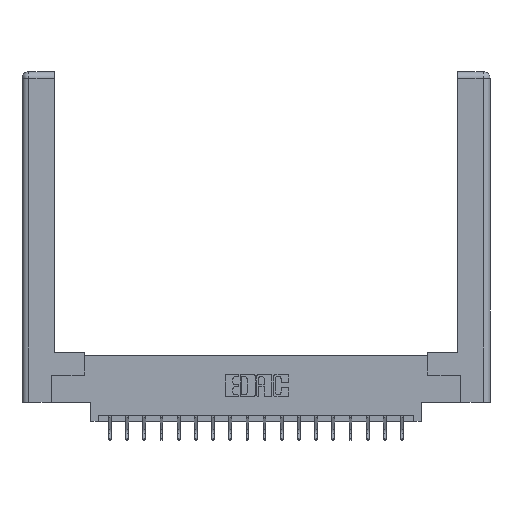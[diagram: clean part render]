
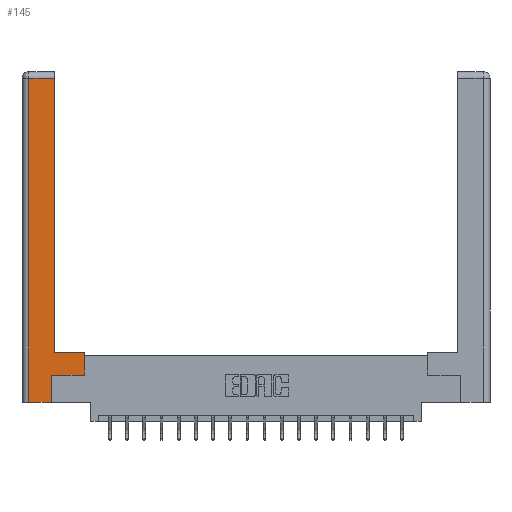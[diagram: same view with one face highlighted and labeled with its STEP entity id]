
A CAD part, top view. The second image highlights one B-rep face of the part: STEP entity #145.
In plain terms, the highlighted planar face has unit normal (0, 0, 1).
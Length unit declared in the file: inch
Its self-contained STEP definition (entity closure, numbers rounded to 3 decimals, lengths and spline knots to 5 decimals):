
#145 = ADVANCED_FACE ( 'NONE', ( #19700 ), #7569, .F. ) ;
#314 = CARTESIAN_POINT ( 'NONE',  ( 0.565, 0.245, 0. ) ) ;
#744 = VECTOR ( 'NONE', #5296, 39.37008 ) ;
#843 = CARTESIAN_POINT ( 'NONE',  ( 0.265, 0., 0. ) ) ;
#1026 = VERTEX_POINT ( 'NONE', #8673 ) ;
#1340 = LINE ( 'NONE', #14225, #16392 ) ;
#1631 = CARTESIAN_POINT ( 'NONE',  ( 0.0615, 2.94, 0. ) ) ;
#2412 = EDGE_CURVE ( 'NONE', #9835, #17495, #4857, .T. ) ;
#2894 = EDGE_CURVE ( 'NONE', #1026, #15038, #7751, .T. ) ;
#3127 = DIRECTION ( 'NONE',  ( -1., 0., 0. ) ) ;
#3463 = CARTESIAN_POINT ( 'NONE',  ( 0.295, 3., 0. ) ) ;
#3524 = DIRECTION ( 'NONE',  ( -1., 0., 0. ) ) ;
#3970 = ORIENTED_EDGE ( 'NONE', *, *, #2412, .T. ) ;
#4178 = ORIENTED_EDGE ( 'NONE', *, *, #19237, .T. ) ;
#4364 = ORIENTED_EDGE ( 'NONE', *, *, #2894, .T. ) ;
#4411 = DIRECTION ( 'NONE',  ( -1., 0., 0. ) ) ;
#4857 = LINE ( 'NONE', #3463, #7535 ) ;
#5009 = ORIENTED_EDGE ( 'NONE', *, *, #16505, .T. ) ;
#5290 = VERTEX_POINT ( 'NONE', #843 ) ;
#5296 = DIRECTION ( 'NONE',  ( 0., -1., 0. ) ) ;
#6194 = ORIENTED_EDGE ( 'NONE', *, *, #15344, .T. ) ;
#6215 = VECTOR ( 'NONE', #14056, 39.37008 ) ;
#6454 = CARTESIAN_POINT ( 'NONE',  ( 0.295, 0.45, 0. ) ) ;
#7167 = ORIENTED_EDGE ( 'NONE', *, *, #18820, .T. ) ;
#7535 = VECTOR ( 'NONE', #15695, 39.37008 ) ;
#7569 = PLANE ( 'NONE',  #8427 ) ;
#7751 = LINE ( 'NONE', #314, #10920 ) ;
#7801 = CARTESIAN_POINT ( 'NONE',  ( 0.265, 0., 0. ) ) ;
#7970 = CARTESIAN_POINT ( 'NONE',  ( 0.565, 0.245, 0. ) ) ;
#8125 = CARTESIAN_POINT ( 'NONE',  ( 0.265, 0.245, 0. ) ) ;
#8427 = AXIS2_PLACEMENT_3D ( 'NONE', #13826, #12539, #3524 ) ;
#8673 = CARTESIAN_POINT ( 'NONE',  ( 0.265, 0.245, 0. ) ) ;
#9017 = LINE ( 'NONE', #13182, #744 ) ;
#9038 = VECTOR ( 'NONE', #4411, 39.37008 ) ;
#9835 = VERTEX_POINT ( 'NONE', #6454 ) ;
#10073 = EDGE_LOOP ( 'NONE', ( #3970, #7167, #6194, #17054, #5009, #4364, #4178, #14923 ) ) ;
#10777 = VERTEX_POINT ( 'NONE', #14488 ) ;
#10828 = DIRECTION ( 'NONE',  ( 0., 1., 0. ) ) ;
#10920 = VECTOR ( 'NONE', #11227, 39.37008 ) ;
#11227 = DIRECTION ( 'NONE',  ( 1., 0., 0. ) ) ;
#11578 = CARTESIAN_POINT ( 'NONE',  ( 0.565, 0.45, 0. ) ) ;
#12539 = DIRECTION ( 'NONE',  ( 0., 0., -1. ) ) ;
#13174 = VERTEX_POINT ( 'NONE', #1631 ) ;
#13182 = CARTESIAN_POINT ( 'NONE',  ( 0.0615, 0., 0. ) ) ;
#13737 = CARTESIAN_POINT ( 'NONE',  ( 0.295, 0.45, 0. ) ) ;
#13826 = CARTESIAN_POINT ( 'NONE',  ( 0., 0., 0. ) ) ;
#14056 = DIRECTION ( 'NONE',  ( 1., 0., 0. ) ) ;
#14225 = CARTESIAN_POINT ( 'NONE',  ( 0.0615, 2.94, 0. ) ) ;
#14488 = CARTESIAN_POINT ( 'NONE',  ( 0.0615, 0., 0. ) ) ;
#14689 = LINE ( 'NONE', #15531, #17329 ) ;
#14914 = EDGE_CURVE ( 'NONE', #19516, #9835, #18420, .T. ) ;
#14923 = ORIENTED_EDGE ( 'NONE', *, *, #14914, .T. ) ;
#15038 = VERTEX_POINT ( 'NONE', #7970 ) ;
#15344 = EDGE_CURVE ( 'NONE', #13174, #10777, #9017, .T. ) ;
#15502 = CARTESIAN_POINT ( 'NONE',  ( 0.295, 2.94, 0. ) ) ;
#15531 = CARTESIAN_POINT ( 'NONE',  ( 0.565, 0.45, 0. ) ) ;
#15695 = DIRECTION ( 'NONE',  ( 0., 1., 0. ) ) ;
#16392 = VECTOR ( 'NONE', #3127, 39.37008 ) ;
#16463 = LINE ( 'NONE', #8125, #17178 ) ;
#16505 = EDGE_CURVE ( 'NONE', #5290, #1026, #16463, .T. ) ;
#16610 = LINE ( 'NONE', #7801, #6215 ) ;
#17054 = ORIENTED_EDGE ( 'NONE', *, *, #18146, .T. ) ;
#17178 = VECTOR ( 'NONE', #17616, 39.37008 ) ;
#17329 = VECTOR ( 'NONE', #10828, 39.37008 ) ;
#17495 = VERTEX_POINT ( 'NONE', #15502 ) ;
#17616 = DIRECTION ( 'NONE',  ( 0., 1., 0. ) ) ;
#18146 = EDGE_CURVE ( 'NONE', #10777, #5290, #16610, .T. ) ;
#18420 = LINE ( 'NONE', #13737, #9038 ) ;
#18820 = EDGE_CURVE ( 'NONE', #17495, #13174, #1340, .T. ) ;
#19237 = EDGE_CURVE ( 'NONE', #15038, #19516, #14689, .T. ) ;
#19516 = VERTEX_POINT ( 'NONE', #11578 ) ;
#19700 = FACE_OUTER_BOUND ( 'NONE', #10073, .T. ) ;
